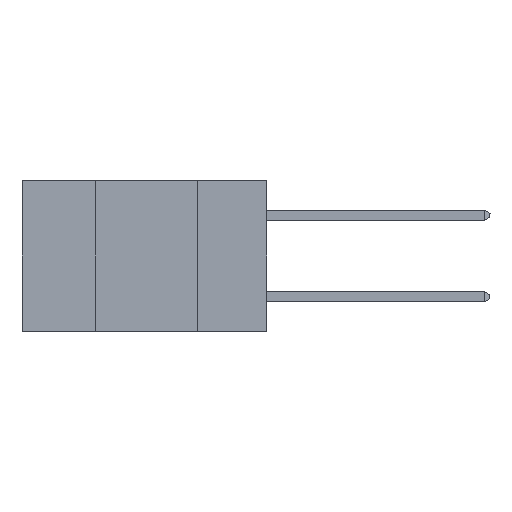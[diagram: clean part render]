
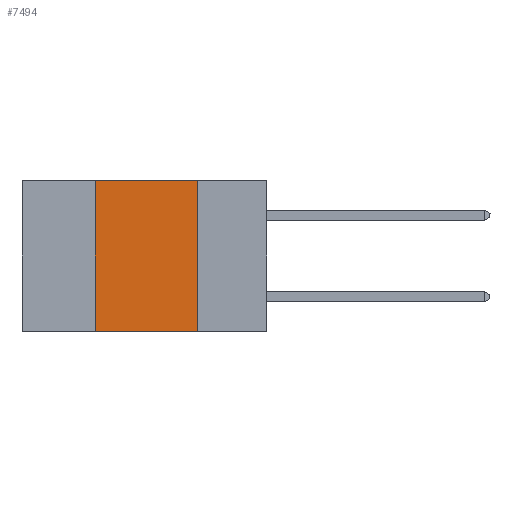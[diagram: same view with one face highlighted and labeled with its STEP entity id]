
A CAD part, left-side view. The second image highlights one B-rep face of the part: STEP entity #7494.
In plain terms, the highlighted planar face has unit normal (-1, 0, 0).
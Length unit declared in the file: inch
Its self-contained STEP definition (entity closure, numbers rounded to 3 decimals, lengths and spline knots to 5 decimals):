
#595 = ORIENTED_EDGE ( 'NONE', *, *, #9044, .F. ) ;
#968 = CARTESIAN_POINT ( 'NONE',  ( 0., 0.42, 0. ) ) ;
#1192 = AXIS2_PLACEMENT_3D ( 'NONE', #7656, #3863, #5559 ) ;
#1751 = ORIENTED_EDGE ( 'NONE', *, *, #8999, .F. ) ;
#1791 = CARTESIAN_POINT ( 'NONE',  ( 0., 0.17, 0. ) ) ;
#2132 = VERTEX_POINT ( 'NONE', #4576 ) ;
#2821 = DIRECTION ( 'NONE',  ( 0., -1., 0. ) ) ;
#3693 = DIRECTION ( 'NONE',  ( 0., 0., -1. ) ) ;
#3863 = DIRECTION ( 'NONE',  ( 1., 0., 0. ) ) ;
#4016 = VERTEX_POINT ( 'NONE', #11383 ) ;
#4333 = FACE_OUTER_BOUND ( 'NONE', #8269, .T. ) ;
#4502 = LINE ( 'NONE', #9272, #10520 ) ;
#4576 = CARTESIAN_POINT ( 'NONE',  ( 0., 0.17, -0.37 ) ) ;
#4724 = VERTEX_POINT ( 'NONE', #7550 ) ;
#4935 = VERTEX_POINT ( 'NONE', #11764 ) ;
#5524 = DIRECTION ( 'NONE',  ( 0., -1., 0. ) ) ;
#5559 = DIRECTION ( 'NONE',  ( 0., 0., -1. ) ) ;
#5851 = CARTESIAN_POINT ( 'NONE',  ( 0., 0.6, 0. ) ) ;
#6047 = ORIENTED_EDGE ( 'NONE', *, *, #6729, .T. ) ;
#6238 = VECTOR ( 'NONE', #3693, 39.37008 ) ;
#6528 = VECTOR ( 'NONE', #8589, 39.37008 ) ;
#6658 = PLANE ( 'NONE',  #1192 ) ;
#6729 = EDGE_CURVE ( 'NONE', #4016, #2132, #4502, .T. ) ;
#7269 = LINE ( 'NONE', #5851, #8592 ) ;
#7494 = ADVANCED_FACE ( 'NONE', ( #4333 ), #6658, .F. ) ;
#7550 = CARTESIAN_POINT ( 'NONE',  ( 0., 0.42, 0. ) ) ;
#7656 = CARTESIAN_POINT ( 'NONE',  ( 0., 0.6, 0. ) ) ;
#8269 = EDGE_LOOP ( 'NONE', ( #1751, #595, #10185, #6047 ) ) ;
#8589 = DIRECTION ( 'NONE',  ( 0., 0., 1. ) ) ;
#8592 = VECTOR ( 'NONE', #2821, 39.37008 ) ;
#8741 = LINE ( 'NONE', #1791, #6238 ) ;
#8999 = EDGE_CURVE ( 'NONE', #4935, #2132, #8741, .T. ) ;
#9044 = EDGE_CURVE ( 'NONE', #4724, #4935, #7269, .T. ) ;
#9138 = EDGE_CURVE ( 'NONE', #4016, #4724, #9473, .T. ) ;
#9272 = CARTESIAN_POINT ( 'NONE',  ( 0., 0.6, -0.37 ) ) ;
#9473 = LINE ( 'NONE', #968, #6528 ) ;
#10185 = ORIENTED_EDGE ( 'NONE', *, *, #9138, .F. ) ;
#10520 = VECTOR ( 'NONE', #5524, 39.37008 ) ;
#11383 = CARTESIAN_POINT ( 'NONE',  ( 0., 0.42, -0.37 ) ) ;
#11764 = CARTESIAN_POINT ( 'NONE',  ( 0., 0.17, 0. ) ) ;
